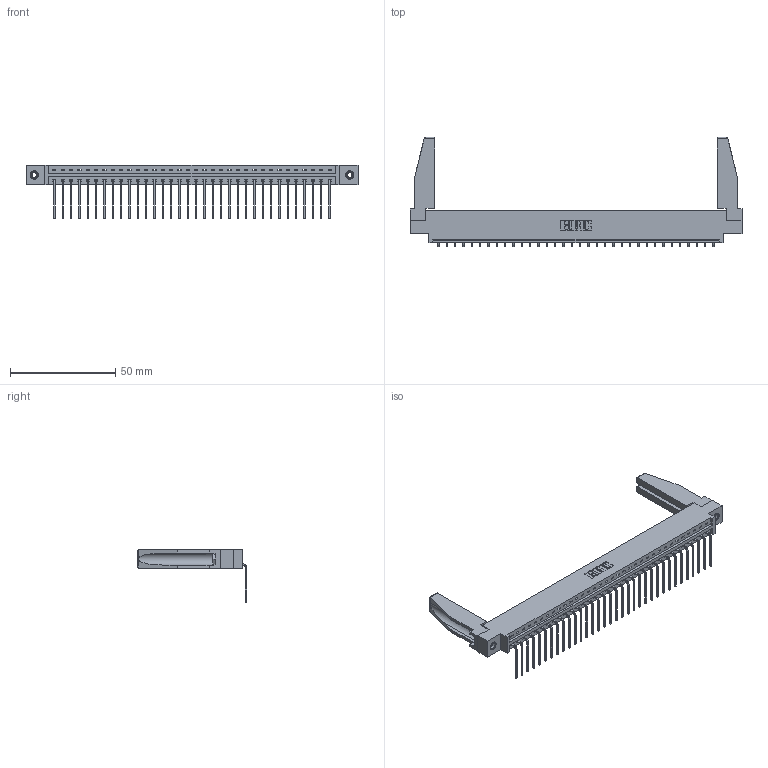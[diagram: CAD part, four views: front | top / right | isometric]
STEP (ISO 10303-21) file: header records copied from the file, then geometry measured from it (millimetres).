
FILE_DESCRIPTION (( 'STEP AP203' ), '1' );
FILE_NAME ('337-034-559-678.STEP', '2019-10-01T12:19:40', ( '' ), ( '' ), 'SwSTEP 2.0', 'SolidWorks 2016', '' );
FILE_SCHEMA (( 'CONFIG_CONTROL_DESIGN' ));
Length unit declared in the file: inch
Products named in the file (5): 337-034-559-678; 307-220-078; 337 Part_0.170 Offset - 0.156 Dia-TI; 345-292-001_558 559 Tail - 1; 345-250-001_345-250-001-102
Assembly tree (39 placements, depth 2):
  337-034-559-678
    337 Part_0.170 Offset - 0.156 Dia-TI
    345-292-001_558 559 Tail - 1  x34
    345-250-001_345-250-001-102  x2
    307-220-078  x2
Bounding box: 157.73 x 51.88 x 25.53 mm (x, y, z)
Volume: 20282.8 mm3; surface area: 21417.6 mm2
Topology: 39 solids, 39 shells, 2424 faces, 7249 edges, 4778 vertices
Faces by surface type: plane 1790, cylinder 618, cone 12, torus 4
Entity records: 28964 total; most frequent: CARTESIAN_POINT 5038, ORIENTED_EDGE 4964, DIRECTION 4266, EDGE_CURVE 2482, VECTOR 2316, LINE 2316, VERTEX_POINT 1648, AXIS2_PLACEMENT_3D 975
